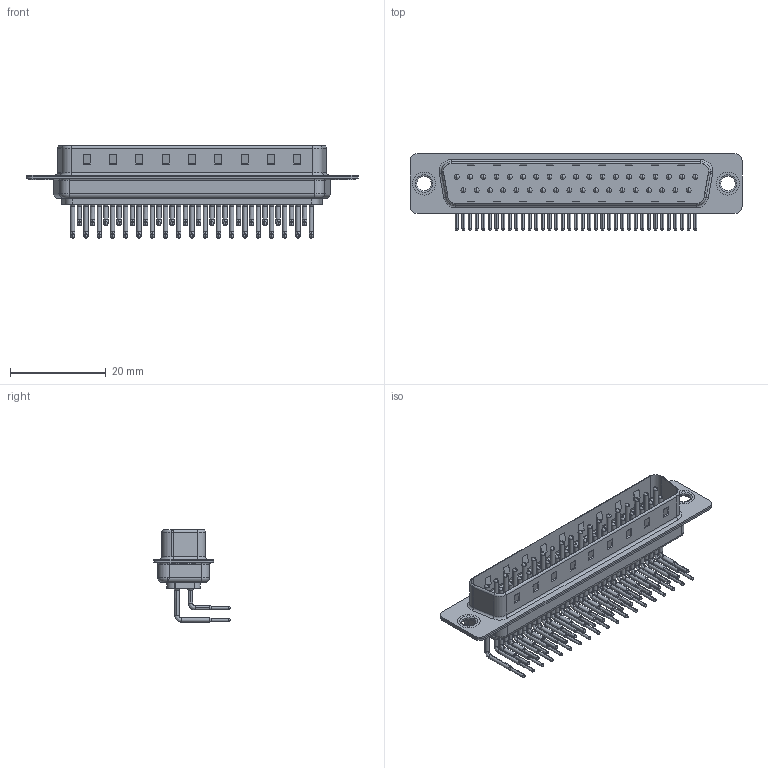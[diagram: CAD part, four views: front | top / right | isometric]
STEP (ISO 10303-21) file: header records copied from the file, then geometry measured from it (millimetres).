
FILE_DESCRIPTION (( 'STEP AP203' ), '1' );
FILE_NAME ('629-M37-340-WN1.STEP', '2018-09-25T21:51:58', ( '' ), ( '' ), 'SwSTEP 2.0', 'SolidWorks 2016', '' );
FILE_SCHEMA (( 'CONFIG_CONTROL_DESIGN' ));
Length unit declared in the file: millimetre
Products named in the file (7): 629M Thru Hole Rivet; 629-M37-340-WN1; 629M Housing_37 Contacts; 629M Shell Front_37 Contacts; 629M Shell Rear_37 Contacts; 629M Contact Row 1; 629M Contact Row 2
Assembly tree (42 placements, depth 2):
  629-M37-340-WN1
    629M Housing_37 Contacts
    629M Shell Front_37 Contacts
    629M Shell Rear_37 Contacts
    629M Contact Row 1  x19
    629M Contact Row 2  x18
    629M Thru Hole Rivet  x2
Bounding box: 69.4 x 16 x 19.29 mm (x, y, z)
Volume: 3972 mm3; surface area: 10469.5 mm2
Topology: 42 solids, 42 shells, 4456 faces, 12483 edges, 8122 vertices
Faces by surface type: plane 2571, cylinder 1457, bspline 222, cone 148, torus 58
Entity records: 28409 total; most frequent: DIRECTION 4857, CARTESIAN_POINT 4746, ORIENTED_EDGE 4358, EDGE_CURVE 2179, AXIS2_PLACEMENT_3D 1794, VERTEX_POINT 1412, LINE 1269, VECTOR 1269
